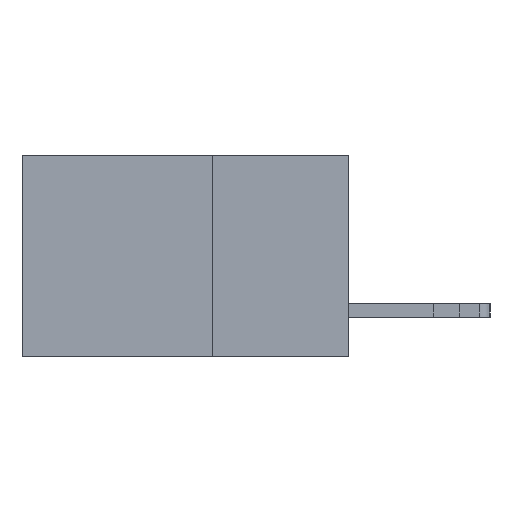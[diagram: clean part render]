
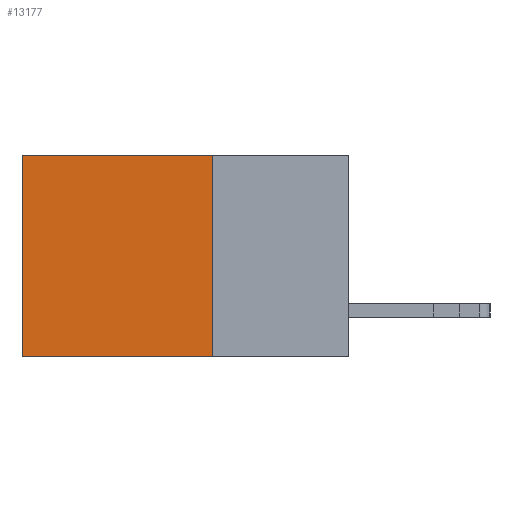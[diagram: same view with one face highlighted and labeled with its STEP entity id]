
A CAD part, left-side view. The second image highlights one B-rep face of the part: STEP entity #13177.
In plain terms, the highlighted planar face has unit normal (-1, 0, 0).
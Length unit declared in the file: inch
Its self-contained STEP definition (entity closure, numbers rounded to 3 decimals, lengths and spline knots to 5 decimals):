
#536 = FACE_OUTER_BOUND ( 'NONE', #5696, .T. ) ;
#1131 = DIRECTION ( 'NONE',  ( 0., 1., 0. ) ) ;
#1935 = EDGE_CURVE ( 'NONE', #5498, #11801, #15140, .T. ) ;
#2216 = VERTEX_POINT ( 'NONE', #9652 ) ;
#2304 = CARTESIAN_POINT ( 'NONE',  ( 0.298, 0.25, 0. ) ) ;
#2368 = CARTESIAN_POINT ( 'NONE',  ( 0.298, 0.25, 0. ) ) ;
#2898 = DIRECTION ( 'NONE',  ( 0., 0., -1. ) ) ;
#3115 = VERTEX_POINT ( 'NONE', #6001 ) ;
#3125 = VECTOR ( 'NONE', #1131, 39.37008 ) ;
#3496 = VECTOR ( 'NONE', #12906, 39.37008 ) ;
#3523 = LINE ( 'NONE', #13018, #3125 ) ;
#3915 = LINE ( 'NONE', #2368, #3496 ) ;
#4018 = AXIS2_PLACEMENT_3D ( 'NONE', #6843, #10817, #2898 ) ;
#4141 = PLANE ( 'NONE',  #4018 ) ;
#4484 = ORIENTED_EDGE ( 'NONE', *, *, #6801, .T. ) ;
#5498 = VERTEX_POINT ( 'NONE', #16490 ) ;
#5696 = EDGE_LOOP ( 'NONE', ( #10510, #12743, #6597, #4484 ) ) ;
#6001 = CARTESIAN_POINT ( 'NONE',  ( 0.298, 0.25, 0. ) ) ;
#6597 = ORIENTED_EDGE ( 'NONE', *, *, #12334, .F. ) ;
#6801 = EDGE_CURVE ( 'NONE', #3115, #5498, #3915, .T. ) ;
#6843 = CARTESIAN_POINT ( 'NONE',  ( 0.298, 0.25, 0. ) ) ;
#7214 = LINE ( 'NONE', #2304, #7622 ) ;
#7622 = VECTOR ( 'NONE', #10239, 39.37008 ) ;
#8212 = VECTOR ( 'NONE', #17004, 39.37008 ) ;
#8984 = CARTESIAN_POINT ( 'NONE',  ( 0.298, 0.6, 0. ) ) ;
#9652 = CARTESIAN_POINT ( 'NONE',  ( 0.298, 0.25, -0.37 ) ) ;
#9851 = EDGE_CURVE ( 'NONE', #2216, #11801, #3523, .T. ) ;
#10239 = DIRECTION ( 'NONE',  ( 0., 0., -1. ) ) ;
#10510 = ORIENTED_EDGE ( 'NONE', *, *, #1935, .T. ) ;
#10817 = DIRECTION ( 'NONE',  ( 1., 0., 0. ) ) ;
#11680 = CARTESIAN_POINT ( 'NONE',  ( 0.298, 0.6, -0.37 ) ) ;
#11801 = VERTEX_POINT ( 'NONE', #11680 ) ;
#12334 = EDGE_CURVE ( 'NONE', #3115, #2216, #7214, .T. ) ;
#12743 = ORIENTED_EDGE ( 'NONE', *, *, #9851, .F. ) ;
#12906 = DIRECTION ( 'NONE',  ( 0., 1., 0. ) ) ;
#13018 = CARTESIAN_POINT ( 'NONE',  ( 0.298, 0.25, -0.37 ) ) ;
#13177 = ADVANCED_FACE ( 'NONE', ( #536 ), #4141, .F. ) ;
#15140 = LINE ( 'NONE', #8984, #8212 ) ;
#16490 = CARTESIAN_POINT ( 'NONE',  ( 0.298, 0.6, 0. ) ) ;
#17004 = DIRECTION ( 'NONE',  ( 0., 0., -1. ) ) ;
